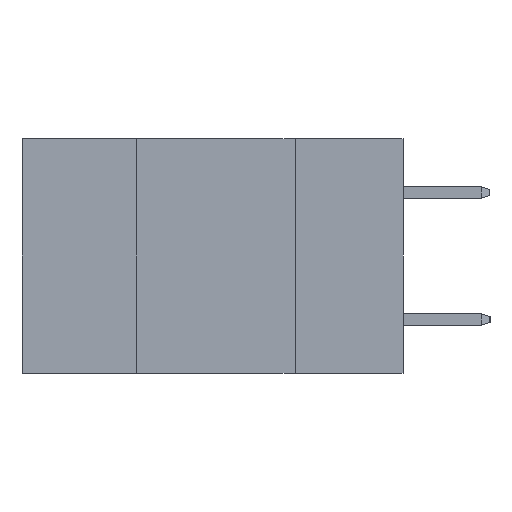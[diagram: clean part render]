
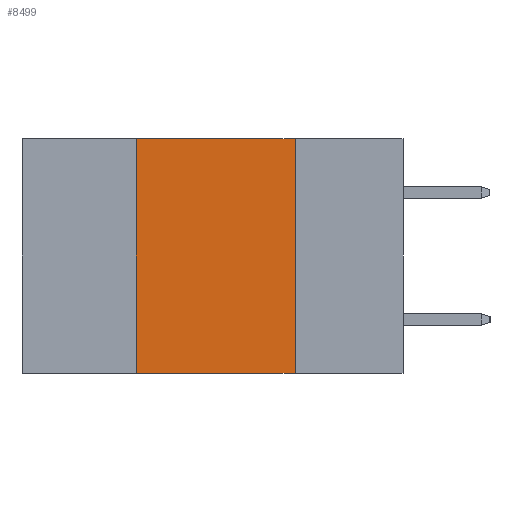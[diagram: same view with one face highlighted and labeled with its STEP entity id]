
A CAD part, left-side view. The second image highlights one B-rep face of the part: STEP entity #8499.
In plain terms, the highlighted planar face has unit normal (-1, 0, 0).
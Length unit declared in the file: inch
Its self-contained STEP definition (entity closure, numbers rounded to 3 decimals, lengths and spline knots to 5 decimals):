
#61 = LINE ( 'NONE', #5814, #5812 ) ;
#529 = DIRECTION ( 'NONE',  ( 0., -1., 0. ) ) ;
#876 = LINE ( 'NONE', #8905, #2874 ) ;
#1160 = FACE_OUTER_BOUND ( 'NONE', #7169, .T. ) ;
#1514 = ORIENTED_EDGE ( 'NONE', *, *, #6475, .F. ) ;
#1520 = LINE ( 'NONE', #2452, #7059 ) ;
#2227 = ORIENTED_EDGE ( 'NONE', *, *, #4164, .F. ) ;
#2452 = CARTESIAN_POINT ( 'NONE',  ( 0., 0.6, 0. ) ) ;
#2874 = VECTOR ( 'NONE', #3228, 39.37008 ) ;
#3084 = DIRECTION ( 'NONE',  ( 0., 0., -1. ) ) ;
#3141 = DIRECTION ( 'NONE',  ( 0., 0., 1. ) ) ;
#3193 = LINE ( 'NONE', #9066, #10859 ) ;
#3228 = DIRECTION ( 'NONE',  ( 0., 0., -1. ) ) ;
#3573 = VERTEX_POINT ( 'NONE', #6658 ) ;
#4000 = CARTESIAN_POINT ( 'NONE',  ( 0., 0.6, 0. ) ) ;
#4164 = EDGE_CURVE ( 'NONE', #3573, #6256, #3193, .T. ) ;
#4958 = VERTEX_POINT ( 'NONE', #10002 ) ;
#5812 = VECTOR ( 'NONE', #6005, 39.37008 ) ;
#5814 = CARTESIAN_POINT ( 'NONE',  ( 0., 0.6, -0.37 ) ) ;
#6005 = DIRECTION ( 'NONE',  ( 0., -1., 0. ) ) ;
#6256 = VERTEX_POINT ( 'NONE', #12798 ) ;
#6475 = EDGE_CURVE ( 'NONE', #4958, #11752, #876, .T. ) ;
#6658 = CARTESIAN_POINT ( 'NONE',  ( 0., 0.42, -0.37 ) ) ;
#7059 = VECTOR ( 'NONE', #529, 39.37008 ) ;
#7169 = EDGE_LOOP ( 'NONE', ( #1514, #11501, #2227, #9655 ) ) ;
#8218 = EDGE_CURVE ( 'NONE', #6256, #4958, #1520, .T. ) ;
#8499 = ADVANCED_FACE ( 'NONE', ( #1160 ), #9202, .F. ) ;
#8877 = EDGE_CURVE ( 'NONE', #3573, #11752, #61, .T. ) ;
#8905 = CARTESIAN_POINT ( 'NONE',  ( 0., 0.17, 0. ) ) ;
#9066 = CARTESIAN_POINT ( 'NONE',  ( 0., 0.42, 0. ) ) ;
#9202 = PLANE ( 'NONE',  #11058 ) ;
#9227 = CARTESIAN_POINT ( 'NONE',  ( 0., 0.17, -0.37 ) ) ;
#9445 = DIRECTION ( 'NONE',  ( 1., 0., 0. ) ) ;
#9655 = ORIENTED_EDGE ( 'NONE', *, *, #8877, .T. ) ;
#10002 = CARTESIAN_POINT ( 'NONE',  ( 0., 0.17, 0. ) ) ;
#10859 = VECTOR ( 'NONE', #3141, 39.37008 ) ;
#11058 = AXIS2_PLACEMENT_3D ( 'NONE', #4000, #9445, #3084 ) ;
#11501 = ORIENTED_EDGE ( 'NONE', *, *, #8218, .F. ) ;
#11752 = VERTEX_POINT ( 'NONE', #9227 ) ;
#12798 = CARTESIAN_POINT ( 'NONE',  ( 0., 0.42, 0. ) ) ;
